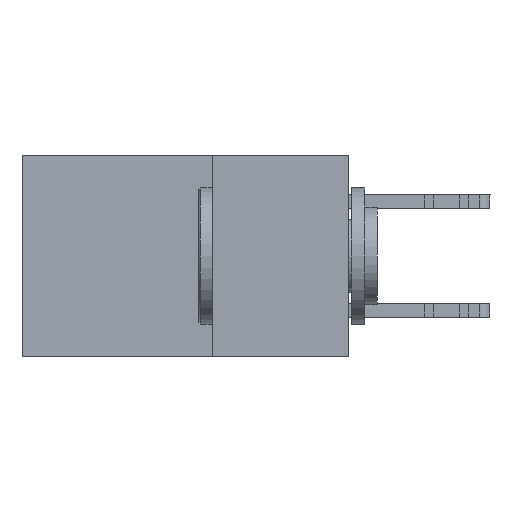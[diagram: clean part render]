
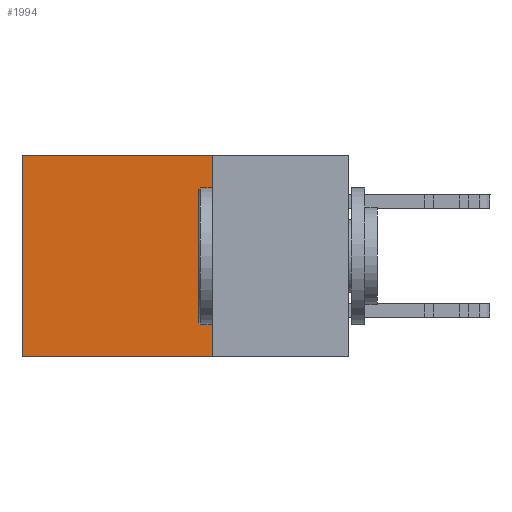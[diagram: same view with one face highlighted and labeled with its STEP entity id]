
A CAD part, left-side view. The second image highlights one B-rep face of the part: STEP entity #1994.
In plain terms, the highlighted planar face has unit normal (-1, 0, 0).
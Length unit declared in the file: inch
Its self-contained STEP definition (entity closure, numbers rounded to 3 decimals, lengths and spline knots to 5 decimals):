
#1073 = EDGE_LOOP ( 'NONE', ( #7289, #26221, #30881, #21757 ) ) ;
#1543 = VECTOR ( 'NONE', #8590, 39.37008 ) ;
#1994 = ADVANCED_FACE ( 'NONE', ( #25561 ), #13225, .F. ) ;
#3324 = EDGE_CURVE ( 'NONE', #7292, #8385, #19178, .T. ) ;
#5627 = LINE ( 'NONE', #25387, #1543 ) ;
#5746 = VERTEX_POINT ( 'NONE', #14961 ) ;
#6519 = AXIS2_PLACEMENT_3D ( 'NONE', #13372, #10597, #20948 ) ;
#6746 = VECTOR ( 'NONE', #9108, 39.37008 ) ;
#7289 = ORIENTED_EDGE ( 'NONE', *, *, #29470, .T. ) ;
#7292 = VERTEX_POINT ( 'NONE', #17804 ) ;
#8385 = VERTEX_POINT ( 'NONE', #14324 ) ;
#8590 = DIRECTION ( 'NONE',  ( 0., 0., -1. ) ) ;
#9108 = DIRECTION ( 'NONE',  ( 0., 0., -1. ) ) ;
#9420 = CARTESIAN_POINT ( 'NONE',  ( 0.298, 0.25, 0. ) ) ;
#10597 = DIRECTION ( 'NONE',  ( 1., 0., 0. ) ) ;
#11758 = CARTESIAN_POINT ( 'NONE',  ( 0.298, 0.25, -0.37 ) ) ;
#11847 = DIRECTION ( 'NONE',  ( 0., 1., 0. ) ) ;
#13225 = PLANE ( 'NONE',  #6519 ) ;
#13372 = CARTESIAN_POINT ( 'NONE',  ( 0.298, 0.25, 0. ) ) ;
#13695 = VECTOR ( 'NONE', #11847, 39.37008 ) ;
#13988 = LINE ( 'NONE', #26509, #13695 ) ;
#14324 = CARTESIAN_POINT ( 'NONE',  ( 0.298, 0.6, -0.37 ) ) ;
#14961 = CARTESIAN_POINT ( 'NONE',  ( 0.298, 0.25, 0. ) ) ;
#15260 = VERTEX_POINT ( 'NONE', #15740 ) ;
#15740 = CARTESIAN_POINT ( 'NONE',  ( 0.298, 0.6, 0. ) ) ;
#17709 = EDGE_CURVE ( 'NONE', #5746, #7292, #31670, .T. ) ;
#17804 = CARTESIAN_POINT ( 'NONE',  ( 0.298, 0.25, -0.37 ) ) ;
#19178 = LINE ( 'NONE', #11758, #29006 ) ;
#20948 = DIRECTION ( 'NONE',  ( 0., 0., -1. ) ) ;
#21757 = ORIENTED_EDGE ( 'NONE', *, *, #23046, .T. ) ;
#23046 = EDGE_CURVE ( 'NONE', #5746, #15260, #13988, .T. ) ;
#25387 = CARTESIAN_POINT ( 'NONE',  ( 0.298, 0.6, 0. ) ) ;
#25561 = FACE_OUTER_BOUND ( 'NONE', #1073, .T. ) ;
#26221 = ORIENTED_EDGE ( 'NONE', *, *, #3324, .F. ) ;
#26509 = CARTESIAN_POINT ( 'NONE',  ( 0.298, 0.25, 0. ) ) ;
#29006 = VECTOR ( 'NONE', #29218, 39.37008 ) ;
#29218 = DIRECTION ( 'NONE',  ( 0., 1., 0. ) ) ;
#29470 = EDGE_CURVE ( 'NONE', #15260, #8385, #5627, .T. ) ;
#30881 = ORIENTED_EDGE ( 'NONE', *, *, #17709, .F. ) ;
#31670 = LINE ( 'NONE', #9420, #6746 ) ;
